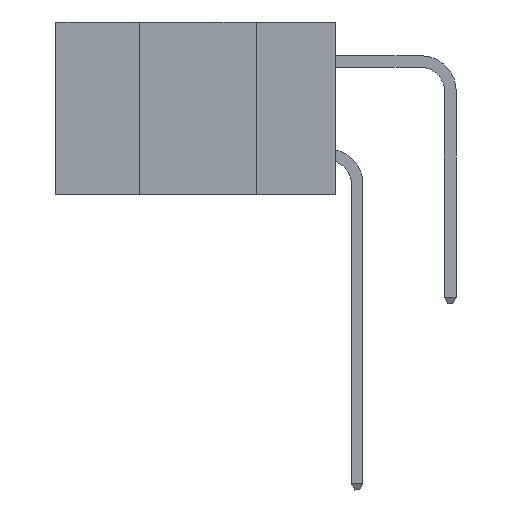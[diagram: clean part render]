
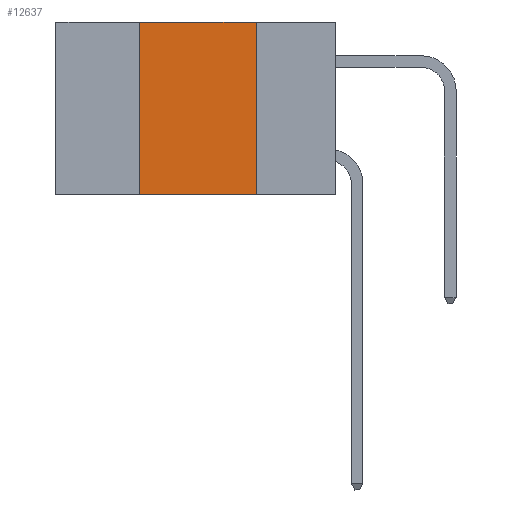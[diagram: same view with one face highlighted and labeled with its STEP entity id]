
A CAD part, left-side view. The second image highlights one B-rep face of the part: STEP entity #12637.
In plain terms, the highlighted planar face has unit normal (-1, 0, 0).
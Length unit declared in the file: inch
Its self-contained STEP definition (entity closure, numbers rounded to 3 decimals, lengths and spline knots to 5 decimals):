
#1504 = DIRECTION ( 'NONE',  ( 0., 0., -1. ) ) ;
#1786 = EDGE_CURVE ( 'NONE', #11526, #3034, #6660, .T. ) ;
#1813 = CARTESIAN_POINT ( 'NONE',  ( 0., 0.6, -0.37 ) ) ;
#2084 = DIRECTION ( 'NONE',  ( 0., 0., 1. ) ) ;
#2796 = LINE ( 'NONE', #3546, #12829 ) ;
#2815 = LINE ( 'NONE', #14951, #12843 ) ;
#3034 = VERTEX_POINT ( 'NONE', #17633 ) ;
#3546 = CARTESIAN_POINT ( 'NONE',  ( 0., 0.17, 0. ) ) ;
#4003 = EDGE_LOOP ( 'NONE', ( #15803, #25466, #22343, #5058 ) ) ;
#4522 = EDGE_CURVE ( 'NONE', #11526, #8688, #13584, .T. ) ;
#5001 = DIRECTION ( 'NONE',  ( 0., -1., 0. ) ) ;
#5058 = ORIENTED_EDGE ( 'NONE', *, *, #4522, .T. ) ;
#6660 = LINE ( 'NONE', #8138, #21787 ) ;
#7546 = CARTESIAN_POINT ( 'NONE',  ( 0., 0.42, -0.37 ) ) ;
#8138 = CARTESIAN_POINT ( 'NONE',  ( 0., 0.42, 0. ) ) ;
#8688 = VERTEX_POINT ( 'NONE', #22553 ) ;
#8984 = VERTEX_POINT ( 'NONE', #23454 ) ;
#11112 = PLANE ( 'NONE',  #25381 ) ;
#11526 = VERTEX_POINT ( 'NONE', #7546 ) ;
#12637 = ADVANCED_FACE ( 'NONE', ( #18677 ), #11112, .F. ) ;
#12829 = VECTOR ( 'NONE', #1504, 39.37008 ) ;
#12843 = VECTOR ( 'NONE', #5001, 39.37008 ) ;
#12974 = VECTOR ( 'NONE', #19563, 39.37008 ) ;
#13111 = DIRECTION ( 'NONE',  ( 0., 0., -1. ) ) ;
#13584 = LINE ( 'NONE', #1813, #12974 ) ;
#14951 = CARTESIAN_POINT ( 'NONE',  ( 0., 0.6, 0. ) ) ;
#15803 = ORIENTED_EDGE ( 'NONE', *, *, #22210, .F. ) ;
#16345 = EDGE_CURVE ( 'NONE', #3034, #8984, #2815, .T. ) ;
#17633 = CARTESIAN_POINT ( 'NONE',  ( 0., 0.42, 0. ) ) ;
#18677 = FACE_OUTER_BOUND ( 'NONE', #4003, .T. ) ;
#19563 = DIRECTION ( 'NONE',  ( 0., -1., 0. ) ) ;
#21787 = VECTOR ( 'NONE', #2084, 39.37008 ) ;
#22210 = EDGE_CURVE ( 'NONE', #8984, #8688, #2796, .T. ) ;
#22343 = ORIENTED_EDGE ( 'NONE', *, *, #1786, .F. ) ;
#22553 = CARTESIAN_POINT ( 'NONE',  ( 0., 0.17, -0.37 ) ) ;
#22848 = CARTESIAN_POINT ( 'NONE',  ( 0., 0.6, 0. ) ) ;
#23454 = CARTESIAN_POINT ( 'NONE',  ( 0., 0.17, 0. ) ) ;
#24754 = DIRECTION ( 'NONE',  ( 1., 0., 0. ) ) ;
#25381 = AXIS2_PLACEMENT_3D ( 'NONE', #22848, #24754, #13111 ) ;
#25466 = ORIENTED_EDGE ( 'NONE', *, *, #16345, .F. ) ;
